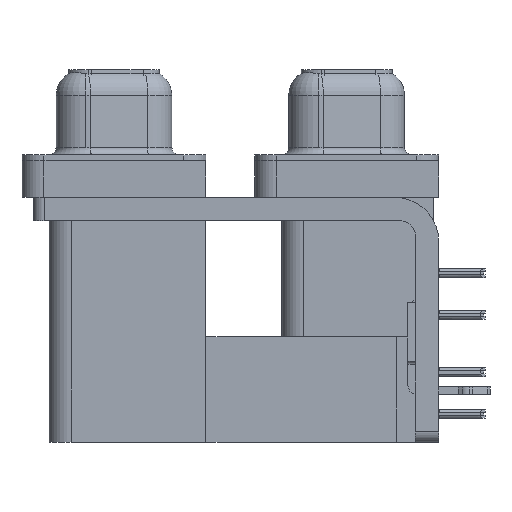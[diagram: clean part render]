
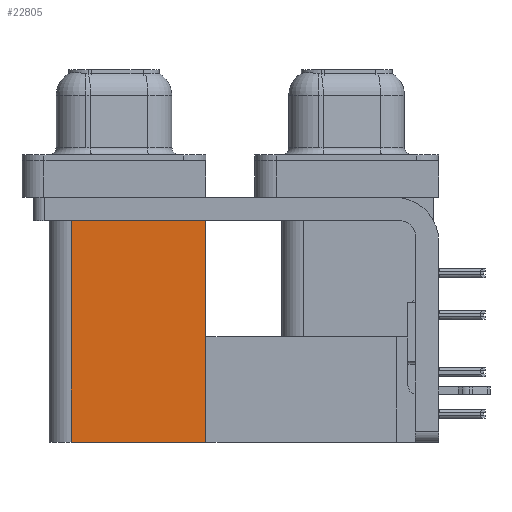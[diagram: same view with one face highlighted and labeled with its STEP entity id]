
A CAD part, left-side view. The second image highlights one B-rep face of the part: STEP entity #22805.
In plain terms, the highlighted planar face has unit normal (-1, 0, 0).
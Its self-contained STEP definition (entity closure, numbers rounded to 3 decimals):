
#348 = CARTESIAN_POINT ( 'NONE',  ( 3.765, 9.6, -2.5 ) ) ;
#3060 = ORIENTED_EDGE ( 'NONE', *, *, #41373, .T. ) ;
#3315 = VECTOR ( 'NONE', #7921, 1000. ) ;
#3504 = FACE_OUTER_BOUND ( 'NONE', #12044, .T. ) ;
#4176 = VERTEX_POINT ( 'NONE', #22795 ) ;
#4874 = EDGE_CURVE ( 'NONE', #4898, #7457, #36419, .T. ) ;
#4898 = VERTEX_POINT ( 'NONE', #31365 ) ;
#6669 = PLANE ( 'NONE',  #15141 ) ;
#7457 = VERTEX_POINT ( 'NONE', #31565 ) ;
#7921 = DIRECTION ( 'NONE',  ( 0., 1., 0. ) ) ;
#8617 = VECTOR ( 'NONE', #38029, 1000. ) ;
#8737 = ORIENTED_EDGE ( 'NONE', *, *, #30920, .F. ) ;
#12044 = EDGE_LOOP ( 'NONE', ( #3060, #33810, #8737, #13211 ) ) ;
#13211 = ORIENTED_EDGE ( 'NONE', *, *, #4874, .T. ) ;
#15141 = AXIS2_PLACEMENT_3D ( 'NONE', #32815, #43591, #18396 ) ;
#15631 = EDGE_CURVE ( 'NONE', #4176, #40826, #23143, .T. ) ;
#18396 = DIRECTION ( 'NONE',  ( 0., 0., -1. ) ) ;
#20146 = CARTESIAN_POINT ( 'NONE',  ( 3.765, 9.6, -19.2 ) ) ;
#22795 = CARTESIAN_POINT ( 'NONE',  ( 3.765, 18.8, -19.2 ) ) ;
#22805 = ADVANCED_FACE ( 'NONE', ( #3504 ), #6669, .F. ) ;
#23143 = LINE ( 'NONE', #29988, #8617 ) ;
#23801 = DIRECTION ( 'NONE',  ( 0., 0., 1. ) ) ;
#27487 = VECTOR ( 'NONE', #33327, 1000. ) ;
#27780 = VECTOR ( 'NONE', #23801, 1000. ) ;
#29988 = CARTESIAN_POINT ( 'NONE',  ( 3.765, 18.8, -19.2 ) ) ;
#30655 = LINE ( 'NONE', #45568, #3315 ) ;
#30920 = EDGE_CURVE ( 'NONE', #4898, #4176, #30655, .T. ) ;
#31365 = CARTESIAN_POINT ( 'NONE',  ( 3.765, 9.6, -19.2 ) ) ;
#31565 = CARTESIAN_POINT ( 'NONE',  ( 3.765, 9.6, -2.5 ) ) ;
#32815 = CARTESIAN_POINT ( 'NONE',  ( 3.765, 9.6, -19.2 ) ) ;
#33327 = DIRECTION ( 'NONE',  ( 0., 1., 0. ) ) ;
#33810 = ORIENTED_EDGE ( 'NONE', *, *, #15631, .F. ) ;
#36419 = LINE ( 'NONE', #20146, #27780 ) ;
#38029 = DIRECTION ( 'NONE',  ( 0., 0., 1. ) ) ;
#40826 = VERTEX_POINT ( 'NONE', #45885 ) ;
#41373 = EDGE_CURVE ( 'NONE', #7457, #40826, #44816, .T. ) ;
#43591 = DIRECTION ( 'NONE',  ( 1., 0., 0. ) ) ;
#44816 = LINE ( 'NONE', #348, #27487 ) ;
#45568 = CARTESIAN_POINT ( 'NONE',  ( 3.765, 9.6, -19.2 ) ) ;
#45885 = CARTESIAN_POINT ( 'NONE',  ( 3.765, 18.8, -2.5 ) ) ;
